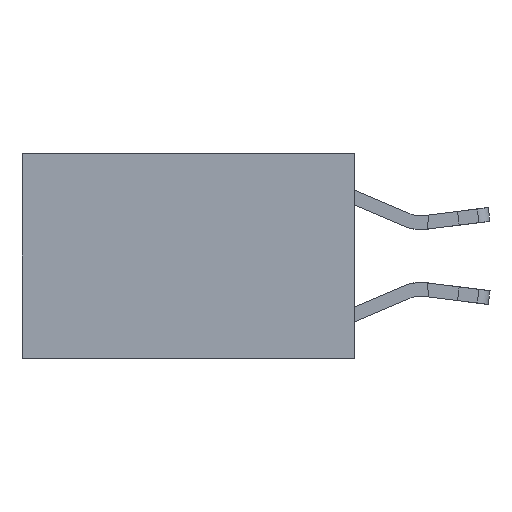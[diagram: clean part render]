
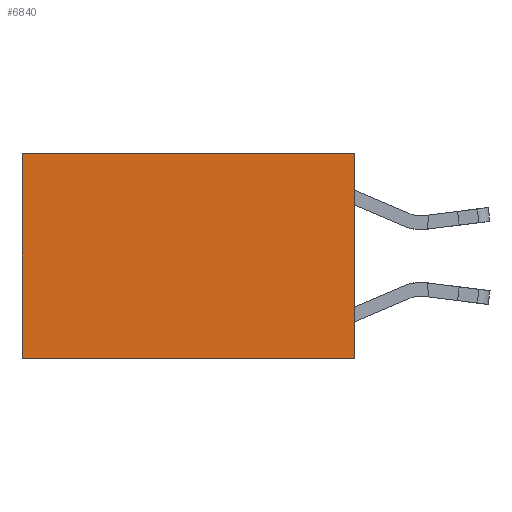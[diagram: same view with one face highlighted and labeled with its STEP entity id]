
A CAD part, left-side view. The second image highlights one B-rep face of the part: STEP entity #6840.
In plain terms, the highlighted planar face has unit normal (-1, 0, 0).
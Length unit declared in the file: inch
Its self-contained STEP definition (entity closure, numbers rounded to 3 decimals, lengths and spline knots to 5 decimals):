
#401 = VERTEX_POINT ( 'NONE', #14239 ) ;
#449 = LINE ( 'NONE', #7370, #18263 ) ;
#937 = DIRECTION ( 'NONE',  ( 0., 0., -1. ) ) ;
#1482 = VECTOR ( 'NONE', #12057, 39.37008 ) ;
#2121 = EDGE_CURVE ( 'NONE', #401, #2452, #13472, .T. ) ;
#2167 = CARTESIAN_POINT ( 'NONE',  ( 0.2625, 0.6, -0.37 ) ) ;
#2371 = DIRECTION ( 'NONE',  ( 0., 0., -1. ) ) ;
#2452 = VERTEX_POINT ( 'NONE', #18124 ) ;
#3025 = CARTESIAN_POINT ( 'NONE',  ( 0.2625, 0., 0. ) ) ;
#3963 = EDGE_CURVE ( 'NONE', #7587, #6717, #17854, .T. ) ;
#6450 = FACE_OUTER_BOUND ( 'NONE', #14270, .T. ) ;
#6566 = VECTOR ( 'NONE', #10223, 39.37008 ) ;
#6717 = VERTEX_POINT ( 'NONE', #2167 ) ;
#6840 = ADVANCED_FACE ( 'NONE', ( #6450 ), #18184, .F. ) ;
#7219 = ORIENTED_EDGE ( 'NONE', *, *, #18536, .T. ) ;
#7370 = CARTESIAN_POINT ( 'NONE',  ( 0.2625, 0., -0.37 ) ) ;
#7587 = VERTEX_POINT ( 'NONE', #17291 ) ;
#8188 = CARTESIAN_POINT ( 'NONE',  ( 0.2625, 0.6, 0. ) ) ;
#9782 = DIRECTION ( 'NONE',  ( 1., 0., 0. ) ) ;
#9956 = ORIENTED_EDGE ( 'NONE', *, *, #3963, .T. ) ;
#10223 = DIRECTION ( 'NONE',  ( 0., 1., 0. ) ) ;
#10640 = CARTESIAN_POINT ( 'NONE',  ( 0.2625, 0., 0. ) ) ;
#10842 = ORIENTED_EDGE ( 'NONE', *, *, #2121, .F. ) ;
#10909 = AXIS2_PLACEMENT_3D ( 'NONE', #11143, #9782, #937 ) ;
#11143 = CARTESIAN_POINT ( 'NONE',  ( 0.2625, 0., 0. ) ) ;
#12057 = DIRECTION ( 'NONE',  ( 0., 0., -1. ) ) ;
#13472 = LINE ( 'NONE', #10640, #1482 ) ;
#13629 = VECTOR ( 'NONE', #2371, 39.37008 ) ;
#14164 = LINE ( 'NONE', #3025, #6566 ) ;
#14239 = CARTESIAN_POINT ( 'NONE',  ( 0.2625, 0., 0. ) ) ;
#14270 = EDGE_LOOP ( 'NONE', ( #9956, #14567, #10842, #7219 ) ) ;
#14535 = DIRECTION ( 'NONE',  ( 0., 1., 0. ) ) ;
#14567 = ORIENTED_EDGE ( 'NONE', *, *, #17704, .F. ) ;
#17291 = CARTESIAN_POINT ( 'NONE',  ( 0.2625, 0.6, 0. ) ) ;
#17704 = EDGE_CURVE ( 'NONE', #2452, #6717, #449, .T. ) ;
#17854 = LINE ( 'NONE', #8188, #13629 ) ;
#18124 = CARTESIAN_POINT ( 'NONE',  ( 0.2625, 0., -0.37 ) ) ;
#18184 = PLANE ( 'NONE',  #10909 ) ;
#18263 = VECTOR ( 'NONE', #14535, 39.37008 ) ;
#18536 = EDGE_CURVE ( 'NONE', #401, #7587, #14164, .T. ) ;
